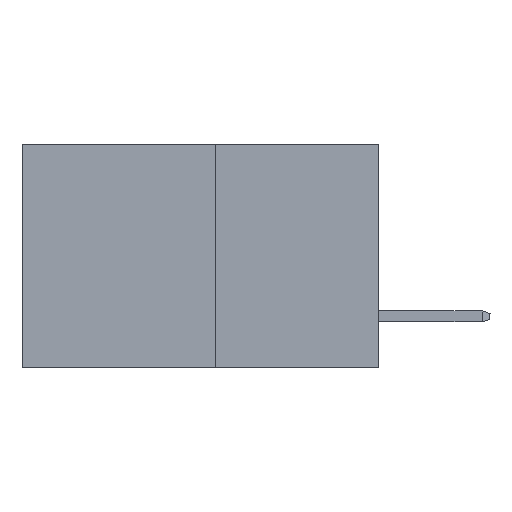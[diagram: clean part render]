
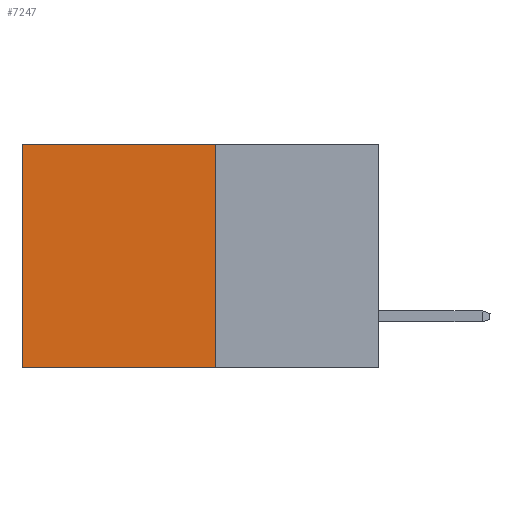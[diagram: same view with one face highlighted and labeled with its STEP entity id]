
A CAD part, left-side view. The second image highlights one B-rep face of the part: STEP entity #7247.
In plain terms, the highlighted planar face has unit normal (-1, 0, 0).
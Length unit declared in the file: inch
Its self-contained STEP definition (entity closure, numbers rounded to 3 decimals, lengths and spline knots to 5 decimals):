
#14 = EDGE_LOOP ( 'NONE', ( #2446, #5582, #8648, #14750 ) ) ;
#906 = LINE ( 'NONE', #8696, #3771 ) ;
#1034 = EDGE_CURVE ( 'NONE', #1449, #5074, #12118, .T. ) ;
#1449 = VERTEX_POINT ( 'NONE', #6241 ) ;
#1528 = DIRECTION ( 'NONE',  ( 0., 0., -1. ) ) ;
#2446 = ORIENTED_EDGE ( 'NONE', *, *, #1034, .T. ) ;
#2834 = LINE ( 'NONE', #13101, #11777 ) ;
#2899 = EDGE_CURVE ( 'NONE', #7233, #1449, #12385, .T. ) ;
#3771 = VECTOR ( 'NONE', #14431, 39.37008 ) ;
#3904 = CARTESIAN_POINT ( 'NONE',  ( 0.277, 0.27, -0.37 ) ) ;
#5074 = VERTEX_POINT ( 'NONE', #14373 ) ;
#5224 = FACE_OUTER_BOUND ( 'NONE', #14, .T. ) ;
#5582 = ORIENTED_EDGE ( 'NONE', *, *, #7206, .F. ) ;
#5592 = VECTOR ( 'NONE', #8842, 39.37008 ) ;
#6241 = CARTESIAN_POINT ( 'NONE',  ( 0.277, 0.59, 0. ) ) ;
#6243 = CARTESIAN_POINT ( 'NONE',  ( 0.277, 0.27, 0. ) ) ;
#6602 = VECTOR ( 'NONE', #15043, 39.37008 ) ;
#7206 = EDGE_CURVE ( 'NONE', #12833, #5074, #2834, .T. ) ;
#7233 = VERTEX_POINT ( 'NONE', #6243 ) ;
#7247 = ADVANCED_FACE ( 'NONE', ( #5224 ), #14298, .F. ) ;
#7338 = EDGE_CURVE ( 'NONE', #7233, #12833, #906, .T. ) ;
#7628 = CARTESIAN_POINT ( 'NONE',  ( 0.277, 0.27, -0.37 ) ) ;
#8551 = DIRECTION ( 'NONE',  ( 1., 0., 0. ) ) ;
#8648 = ORIENTED_EDGE ( 'NONE', *, *, #7338, .F. ) ;
#8696 = CARTESIAN_POINT ( 'NONE',  ( 0.277, 0.27, -0.37 ) ) ;
#8842 = DIRECTION ( 'NONE',  ( 0., 0., -1. ) ) ;
#11777 = VECTOR ( 'NONE', #14244, 39.37008 ) ;
#12118 = LINE ( 'NONE', #12772, #5592 ) ;
#12385 = LINE ( 'NONE', #14919, #6602 ) ;
#12772 = CARTESIAN_POINT ( 'NONE',  ( 0.277, 0.59, -0.37 ) ) ;
#12833 = VERTEX_POINT ( 'NONE', #7628 ) ;
#13101 = CARTESIAN_POINT ( 'NONE',  ( 0.277, 0.27, -0.37 ) ) ;
#14196 = AXIS2_PLACEMENT_3D ( 'NONE', #3904, #8551, #1528 ) ;
#14244 = DIRECTION ( 'NONE',  ( 0., 1., 0. ) ) ;
#14298 = PLANE ( 'NONE',  #14196 ) ;
#14373 = CARTESIAN_POINT ( 'NONE',  ( 0.277, 0.59, -0.37 ) ) ;
#14431 = DIRECTION ( 'NONE',  ( 0., 0., -1. ) ) ;
#14750 = ORIENTED_EDGE ( 'NONE', *, *, #2899, .T. ) ;
#14919 = CARTESIAN_POINT ( 'NONE',  ( 0.277, 0.27, 0. ) ) ;
#15043 = DIRECTION ( 'NONE',  ( 0., 1., 0. ) ) ;
